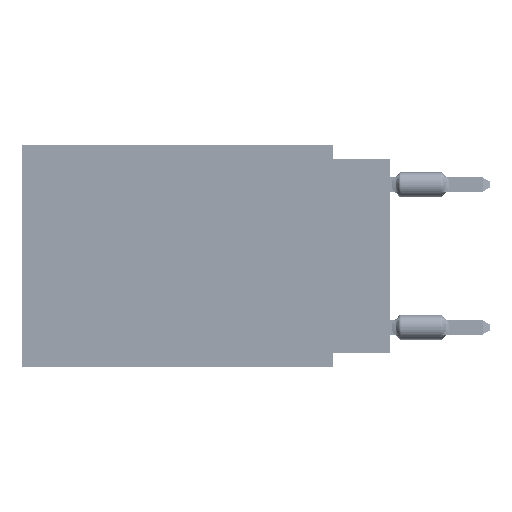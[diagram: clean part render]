
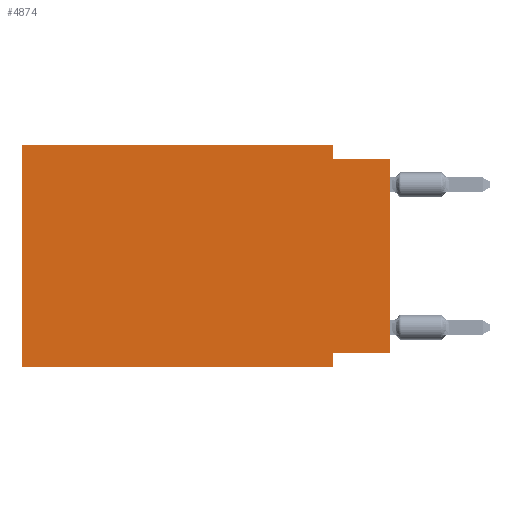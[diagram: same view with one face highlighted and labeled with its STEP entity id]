
A CAD part, left-side view. The second image highlights one B-rep face of the part: STEP entity #4874.
In plain terms, the highlighted planar face has unit normal (-1, 0, 0).
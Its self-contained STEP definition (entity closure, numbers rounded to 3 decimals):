
#762 = EDGE_CURVE ( 'NONE', #40741, #44204, #74896, .T. ) ;
#1169 = EDGE_CURVE ( 'NONE', #14837, #6645, #31699, .T. ) ;
#2259 = LINE ( 'NONE', #77728, #39569 ) ;
#4874 = ADVANCED_FACE ( 'NONE', ( #35787 ), #36192, .F. ) ;
#5602 = LINE ( 'NONE', #12506, #28084 ) ;
#6232 = VECTOR ( 'NONE', #11065, 1000. ) ;
#6645 = VERTEX_POINT ( 'NONE', #13779 ) ;
#9151 = DIRECTION ( 'NONE',  ( 0., 0., -1. ) ) ;
#9367 = EDGE_CURVE ( 'NONE', #44204, #22747, #2259, .T. ) ;
#10864 = CARTESIAN_POINT ( 'NONE',  ( 0., 16.383, -9.906 ) ) ;
#11065 = DIRECTION ( 'NONE',  ( 0., -1., 0. ) ) ;
#12506 = CARTESIAN_POINT ( 'NONE',  ( 0., 0., 0. ) ) ;
#13650 = CARTESIAN_POINT ( 'NONE',  ( 0., 2.54, -9.906 ) ) ;
#13779 = CARTESIAN_POINT ( 'NONE',  ( 0., 2.54, 0. ) ) ;
#14024 = ORIENTED_EDGE ( 'NONE', *, *, #26146, .T. ) ;
#14097 = VECTOR ( 'NONE', #74328, 1000. ) ;
#14335 = CARTESIAN_POINT ( 'NONE',  ( 0., 16.383, -9.906 ) ) ;
#14837 = VERTEX_POINT ( 'NONE', #69669 ) ;
#15365 = VECTOR ( 'NONE', #29950, 1000. ) ;
#16800 = VECTOR ( 'NONE', #79088, 1000. ) ;
#16980 = CARTESIAN_POINT ( 'NONE',  ( 0., 0., -9.271 ) ) ;
#22747 = VERTEX_POINT ( 'NONE', #13650 ) ;
#23872 = CARTESIAN_POINT ( 'NONE',  ( 0., 16.383, 0. ) ) ;
#25985 = CARTESIAN_POINT ( 'NONE',  ( 0., 2.54, -9.271 ) ) ;
#26146 = EDGE_CURVE ( 'NONE', #47570, #22747, #79430, .T. ) ;
#26606 = VERTEX_POINT ( 'NONE', #40780 ) ;
#28084 = VECTOR ( 'NONE', #37239, 1000. ) ;
#28742 = ORIENTED_EDGE ( 'NONE', *, *, #1169, .F. ) ;
#29189 = ORIENTED_EDGE ( 'NONE', *, *, #9367, .F. ) ;
#29950 = DIRECTION ( 'NONE',  ( 0., 1., 0. ) ) ;
#30510 = CARTESIAN_POINT ( 'NONE',  ( 0., 0., -0.635 ) ) ;
#31699 = LINE ( 'NONE', #61358, #14097 ) ;
#32013 = EDGE_CURVE ( 'NONE', #47570, #14837, #72992, .T. ) ;
#33133 = VECTOR ( 'NONE', #75732, 1000. ) ;
#35787 = FACE_OUTER_BOUND ( 'NONE', #55636, .T. ) ;
#36192 = PLANE ( 'NONE',  #38920 ) ;
#37239 = DIRECTION ( 'NONE',  ( 0., 0., 1. ) ) ;
#37786 = VECTOR ( 'NONE', #66066, 1000. ) ;
#38739 = ORIENTED_EDGE ( 'NONE', *, *, #32013, .F. ) ;
#38788 = CARTESIAN_POINT ( 'NONE',  ( 0., 2.54, 0. ) ) ;
#38920 = AXIS2_PLACEMENT_3D ( 'NONE', #59365, #48348, #79619 ) ;
#39569 = VECTOR ( 'NONE', #9151, 1000. ) ;
#40741 = VERTEX_POINT ( 'NONE', #48893 ) ;
#40780 = CARTESIAN_POINT ( 'NONE',  ( 0., 2.54, -0.635 ) ) ;
#44064 = LINE ( 'NONE', #38788, #33133 ) ;
#44204 = VERTEX_POINT ( 'NONE', #25985 ) ;
#47173 = VERTEX_POINT ( 'NONE', #48703 ) ;
#47570 = VERTEX_POINT ( 'NONE', #14335 ) ;
#48348 = DIRECTION ( 'NONE',  ( 1., 0., 0. ) ) ;
#48703 = CARTESIAN_POINT ( 'NONE',  ( 0., 0., -0.635 ) ) ;
#48893 = CARTESIAN_POINT ( 'NONE',  ( 0., 0., -9.271 ) ) ;
#50162 = ORIENTED_EDGE ( 'NONE', *, *, #762, .F. ) ;
#51236 = ORIENTED_EDGE ( 'NONE', *, *, #58078, .F. ) ;
#51562 = EDGE_CURVE ( 'NONE', #40741, #47173, #5602, .T. ) ;
#53271 = EDGE_CURVE ( 'NONE', #26606, #47173, #60980, .T. ) ;
#54862 = ORIENTED_EDGE ( 'NONE', *, *, #53271, .F. ) ;
#55636 = EDGE_LOOP ( 'NONE', ( #75362, #54862, #51236, #28742, #38739, #14024, #29189, #50162 ) ) ;
#58078 = EDGE_CURVE ( 'NONE', #6645, #26606, #44064, .T. ) ;
#59365 = CARTESIAN_POINT ( 'NONE',  ( 0., 16.383, 0. ) ) ;
#60980 = LINE ( 'NONE', #30510, #6232 ) ;
#61358 = CARTESIAN_POINT ( 'NONE',  ( 0., 16.383, 0. ) ) ;
#66066 = DIRECTION ( 'NONE',  ( 0., -1., 0. ) ) ;
#69669 = CARTESIAN_POINT ( 'NONE',  ( 0., 16.383, 0. ) ) ;
#72992 = LINE ( 'NONE', #23872, #16800 ) ;
#74328 = DIRECTION ( 'NONE',  ( 0., -1., 0. ) ) ;
#74896 = LINE ( 'NONE', #16980, #15365 ) ;
#75362 = ORIENTED_EDGE ( 'NONE', *, *, #51562, .T. ) ;
#75732 = DIRECTION ( 'NONE',  ( 0., 0., -1. ) ) ;
#77728 = CARTESIAN_POINT ( 'NONE',  ( 0., 2.54, -9.906 ) ) ;
#79088 = DIRECTION ( 'NONE',  ( 0., 0., 1. ) ) ;
#79430 = LINE ( 'NONE', #10864, #37786 ) ;
#79619 = DIRECTION ( 'NONE',  ( 0., 0., -1. ) ) ;
